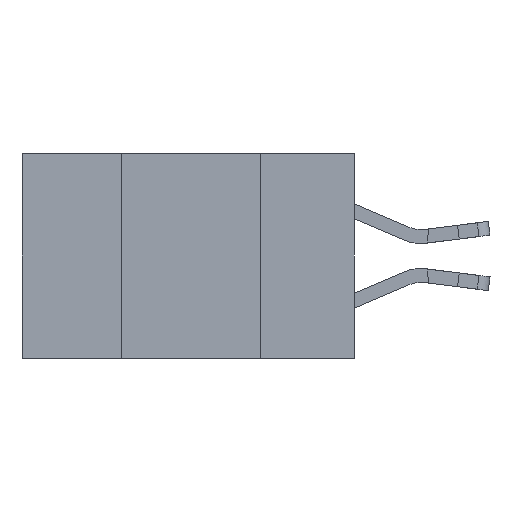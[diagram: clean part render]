
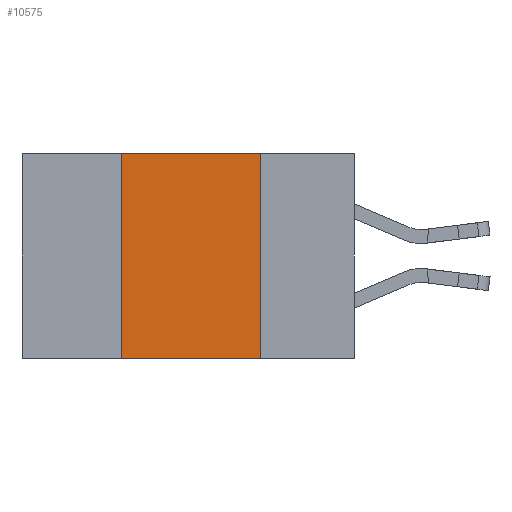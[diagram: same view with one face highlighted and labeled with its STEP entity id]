
A CAD part, left-side view. The second image highlights one B-rep face of the part: STEP entity #10575.
In plain terms, the highlighted planar face has unit normal (-1, 0, 0).
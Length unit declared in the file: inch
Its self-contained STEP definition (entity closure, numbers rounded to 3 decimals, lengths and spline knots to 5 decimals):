
#129 = CARTESIAN_POINT ( 'NONE',  ( 0., 0.42, -0.37 ) ) ;
#521 = DIRECTION ( 'NONE',  ( 0., -1., 0. ) ) ;
#764 = CARTESIAN_POINT ( 'NONE',  ( 0., 0.6, -0.37 ) ) ;
#849 = VECTOR ( 'NONE', #2890, 39.37008 ) ;
#1253 = PLANE ( 'NONE',  #9934 ) ;
#1956 = CARTESIAN_POINT ( 'NONE',  ( 0., 0.6, 0. ) ) ;
#2237 = CARTESIAN_POINT ( 'NONE',  ( 0., 0.17, 0. ) ) ;
#2320 = DIRECTION ( 'NONE',  ( 0., 0., -1. ) ) ;
#2467 = ORIENTED_EDGE ( 'NONE', *, *, #3425, .F. ) ;
#2578 = LINE ( 'NONE', #1956, #12560 ) ;
#2742 = VERTEX_POINT ( 'NONE', #8275 ) ;
#2890 = DIRECTION ( 'NONE',  ( 0., 0., -1. ) ) ;
#2941 = CARTESIAN_POINT ( 'NONE',  ( 0., 0.17, -0.37 ) ) ;
#3425 = EDGE_CURVE ( 'NONE', #9858, #2742, #6654, .T. ) ;
#3499 = ORIENTED_EDGE ( 'NONE', *, *, #4299, .F. ) ;
#3588 = EDGE_CURVE ( 'NONE', #6423, #2742, #6491, .T. ) ;
#3824 = VECTOR ( 'NONE', #521, 39.37008 ) ;
#4299 = EDGE_CURVE ( 'NONE', #6423, #12583, #10593, .T. ) ;
#4585 = CARTESIAN_POINT ( 'NONE',  ( 0., 0.42, -0.37 ) ) ;
#6398 = CARTESIAN_POINT ( 'NONE',  ( 0., 0.6, 0. ) ) ;
#6423 = VERTEX_POINT ( 'NONE', #129 ) ;
#6491 = LINE ( 'NONE', #764, #3824 ) ;
#6556 = DIRECTION ( 'NONE',  ( 0., 0., 1. ) ) ;
#6654 = LINE ( 'NONE', #2941, #849 ) ;
#6855 = EDGE_CURVE ( 'NONE', #12583, #9858, #2578, .T. ) ;
#8120 = VECTOR ( 'NONE', #6556, 39.37008 ) ;
#8275 = CARTESIAN_POINT ( 'NONE',  ( 0., 0.17, -0.37 ) ) ;
#8326 = DIRECTION ( 'NONE',  ( 1., 0., 0. ) ) ;
#8684 = EDGE_LOOP ( 'NONE', ( #2467, #10597, #3499, #11741 ) ) ;
#9351 = CARTESIAN_POINT ( 'NONE',  ( 0., 0.42, 0. ) ) ;
#9858 = VERTEX_POINT ( 'NONE', #2237 ) ;
#9934 = AXIS2_PLACEMENT_3D ( 'NONE', #6398, #8326, #2320 ) ;
#10448 = FACE_OUTER_BOUND ( 'NONE', #8684, .T. ) ;
#10575 = ADVANCED_FACE ( 'NONE', ( #10448 ), #1253, .F. ) ;
#10593 = LINE ( 'NONE', #4585, #8120 ) ;
#10597 = ORIENTED_EDGE ( 'NONE', *, *, #6855, .F. ) ;
#10830 = DIRECTION ( 'NONE',  ( 0., -1., 0. ) ) ;
#11741 = ORIENTED_EDGE ( 'NONE', *, *, #3588, .T. ) ;
#12560 = VECTOR ( 'NONE', #10830, 39.37008 ) ;
#12583 = VERTEX_POINT ( 'NONE', #9351 ) ;
